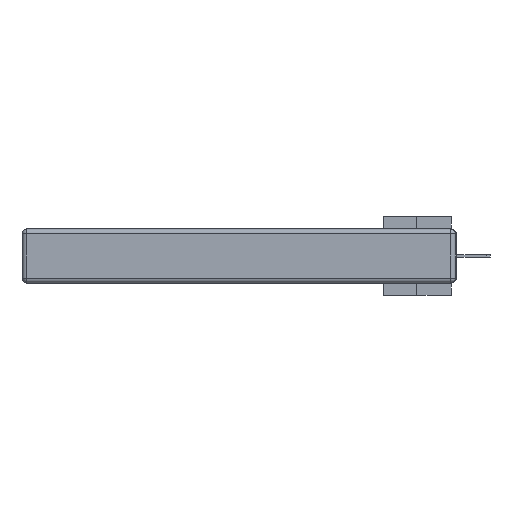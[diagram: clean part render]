
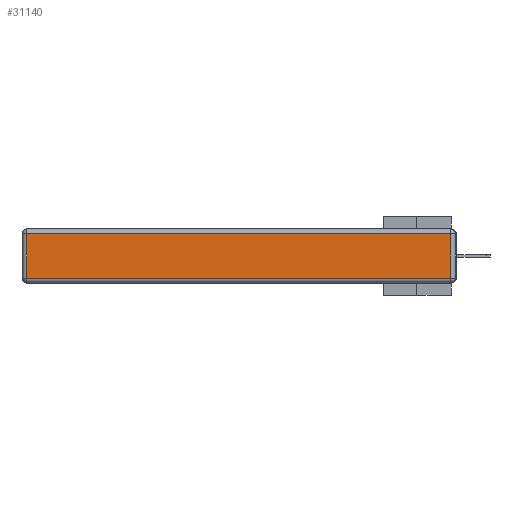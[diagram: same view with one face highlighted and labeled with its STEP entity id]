
A CAD part, left-side view. The second image highlights one B-rep face of the part: STEP entity #31140.
In plain terms, the highlighted planar face has unit normal (-1, 0, 0).
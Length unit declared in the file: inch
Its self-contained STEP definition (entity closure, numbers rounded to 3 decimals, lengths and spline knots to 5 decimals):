
#831 = DIRECTION ( 'NONE',  ( -1., 0., 0. ) ) ;
#1045 = VERTEX_POINT ( 'NONE', #22926 ) ;
#1714 = DIRECTION ( 'NONE',  ( 0., 0., 1. ) ) ;
#2008 = CARTESIAN_POINT ( 'NONE',  ( 0., 0.03, -0.03 ) ) ;
#3049 = CARTESIAN_POINT ( 'NONE',  ( 0., 2.72, -0.343 ) ) ;
#5617 = DIRECTION ( 'NONE',  ( 0., 0., -1. ) ) ;
#6450 = ORIENTED_EDGE ( 'NONE', *, *, #14224, .T. ) ;
#7826 = ORIENTED_EDGE ( 'NONE', *, *, #29481, .T. ) ;
#8417 = DIRECTION ( 'NONE',  ( 0., 1., 0. ) ) ;
#9454 = VERTEX_POINT ( 'NONE', #29251 ) ;
#11020 = CARTESIAN_POINT ( 'NONE',  ( 0., 2.75, -0.03 ) ) ;
#11515 = LINE ( 'NONE', #14175, #24265 ) ;
#12494 = EDGE_CURVE ( 'NONE', #30306, #1045, #15041, .T. ) ;
#13371 = ORIENTED_EDGE ( 'NONE', *, *, #12494, .T. ) ;
#14175 = CARTESIAN_POINT ( 'NONE',  ( 0., 0., -0.313 ) ) ;
#14224 = EDGE_CURVE ( 'NONE', #18095, #30306, #30485, .T. ) ;
#14726 = ORIENTED_EDGE ( 'NONE', *, *, #27804, .T. ) ;
#15041 = LINE ( 'NONE', #3049, #27726 ) ;
#16302 = CARTESIAN_POINT ( 'NONE',  ( 0., 0., -0.343 ) ) ;
#16764 = DIRECTION ( 'NONE',  ( 0., -1., 0. ) ) ;
#17101 = VECTOR ( 'NONE', #8417, 39.37008 ) ;
#18095 = VERTEX_POINT ( 'NONE', #2008 ) ;
#18893 = DIRECTION ( 'NONE',  ( 0., 0., 1. ) ) ;
#21304 = PLANE ( 'NONE',  #25304 ) ;
#22926 = CARTESIAN_POINT ( 'NONE',  ( 0., 2.72, -0.313 ) ) ;
#24265 = VECTOR ( 'NONE', #16764, 39.37008 ) ;
#24700 = CARTESIAN_POINT ( 'NONE',  ( 0., 0.03, -0.343 ) ) ;
#25304 = AXIS2_PLACEMENT_3D ( 'NONE', #16302, #831, #18893 ) ;
#25974 = VECTOR ( 'NONE', #1714, 39.37008 ) ;
#26160 = FACE_OUTER_BOUND ( 'NONE', #28551, .T. ) ;
#27726 = VECTOR ( 'NONE', #5617, 39.37008 ) ;
#27804 = EDGE_CURVE ( 'NONE', #9454, #18095, #31076, .T. ) ;
#28551 = EDGE_LOOP ( 'NONE', ( #7826, #14726, #6450, #13371 ) ) ;
#29251 = CARTESIAN_POINT ( 'NONE',  ( 0., 0.03, -0.313 ) ) ;
#29481 = EDGE_CURVE ( 'NONE', #1045, #9454, #11515, .T. ) ;
#30306 = VERTEX_POINT ( 'NONE', #30473 ) ;
#30473 = CARTESIAN_POINT ( 'NONE',  ( 0., 2.72, -0.03 ) ) ;
#30485 = LINE ( 'NONE', #11020, #17101 ) ;
#31076 = LINE ( 'NONE', #24700, #25974 ) ;
#31140 = ADVANCED_FACE ( 'NONE', ( #26160 ), #21304, .T. ) ;
